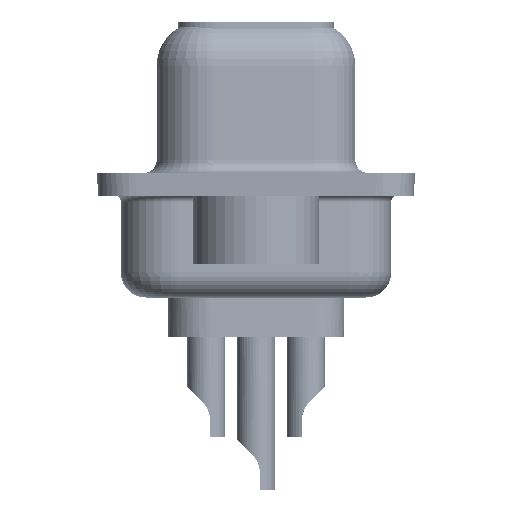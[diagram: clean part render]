
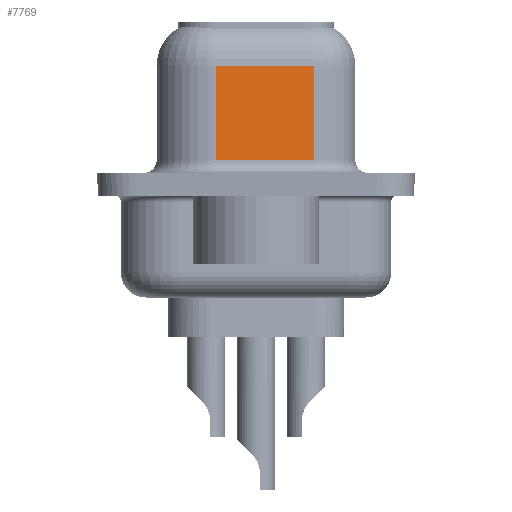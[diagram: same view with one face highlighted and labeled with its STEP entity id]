
A CAD part, left-side view. The second image highlights one B-rep face of the part: STEP entity #7769.
In plain terms, the highlighted planar face has unit normal (-0.985, -0.174, 0).
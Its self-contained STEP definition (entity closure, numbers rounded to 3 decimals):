
#407 = DIRECTION ( 'NONE',  ( 0.174, -0.985, 0. ) ) ;
#1051 = LINE ( 'NONE', #4329, #11509 ) ;
#3317 = CARTESIAN_POINT ( 'NONE',  ( 4.38, 1.603, 6.45 ) ) ;
#3739 = LINE ( 'NONE', #3317, #26372 ) ;
#3931 = FACE_OUTER_BOUND ( 'NONE', #9187, .T. ) ;
#3987 = VECTOR ( 'NONE', #4639, 1000. ) ;
#4329 = CARTESIAN_POINT ( 'NONE',  ( 5.068, -2.297, 6.45 ) ) ;
#4639 = DIRECTION ( 'NONE',  ( -0.174, 0.985, 0. ) ) ;
#7769 = ADVANCED_FACE ( 'NONE', ( #3931 ), #20773, .F. ) ;
#9187 = EDGE_LOOP ( 'NONE', ( #35583, #42373, #17828, #14077 ) ) ;
#11509 = VECTOR ( 'NONE', #41347, 1000. ) ;
#12115 = VERTEX_POINT ( 'NONE', #31083 ) ;
#13305 = CARTESIAN_POINT ( 'NONE',  ( 4.38, 1.603, 0.95 ) ) ;
#13534 = LINE ( 'NONE', #23626, #14628 ) ;
#14077 = ORIENTED_EDGE ( 'NONE', *, *, #14948, .T. ) ;
#14628 = VECTOR ( 'NONE', #407, 1000. ) ;
#14948 = EDGE_CURVE ( 'NONE', #39462, #16887, #13534, .T. ) ;
#15624 = VERTEX_POINT ( 'NONE', #30779 ) ;
#16887 = VERTEX_POINT ( 'NONE', #30195 ) ;
#17755 = CARTESIAN_POINT ( 'NONE',  ( 5.068, -2.297, 4.7 ) ) ;
#17828 = ORIENTED_EDGE ( 'NONE', *, *, #24548, .T. ) ;
#20773 = PLANE ( 'NONE',  #34542 ) ;
#23626 = CARTESIAN_POINT ( 'NONE',  ( 5.068, -2.297, 0.95 ) ) ;
#24548 = EDGE_CURVE ( 'NONE', #15624, #39462, #3739, .T. ) ;
#26372 = VECTOR ( 'NONE', #30454, 1000. ) ;
#27152 = DIRECTION ( 'NONE',  ( -0.174, 0.985, 0. ) ) ;
#30195 = CARTESIAN_POINT ( 'NONE',  ( 5.068, -2.297, 0.95 ) ) ;
#30454 = DIRECTION ( 'NONE',  ( 0., 0., -1. ) ) ;
#30779 = CARTESIAN_POINT ( 'NONE',  ( 4.38, 1.603, 4.7 ) ) ;
#31083 = CARTESIAN_POINT ( 'NONE',  ( 5.068, -2.297, 4.7 ) ) ;
#34287 = EDGE_CURVE ( 'NONE', #12115, #15624, #41013, .T. ) ;
#34542 = AXIS2_PLACEMENT_3D ( 'NONE', #37858, #41376, #27152 ) ;
#35583 = ORIENTED_EDGE ( 'NONE', *, *, #38279, .F. ) ;
#37858 = CARTESIAN_POINT ( 'NONE',  ( 5.068, -2.297, 6.45 ) ) ;
#38279 = EDGE_CURVE ( 'NONE', #12115, #16887, #1051, .T. ) ;
#39462 = VERTEX_POINT ( 'NONE', #13305 ) ;
#41013 = LINE ( 'NONE', #17755, #3987 ) ;
#41347 = DIRECTION ( 'NONE',  ( 0., 0., -1. ) ) ;
#41376 = DIRECTION ( 'NONE',  ( 0.985, 0.174, 0. ) ) ;
#42373 = ORIENTED_EDGE ( 'NONE', *, *, #34287, .T. ) ;
